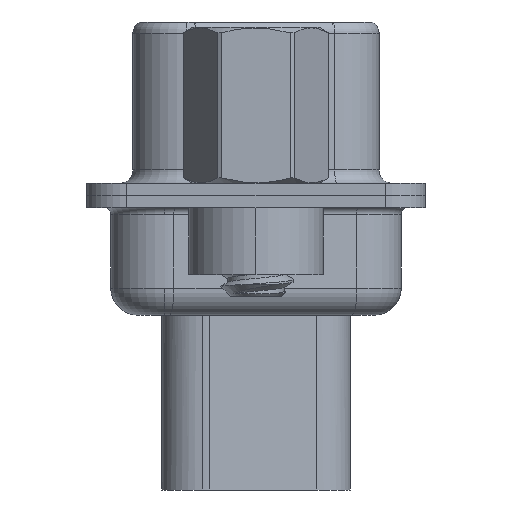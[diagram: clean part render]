
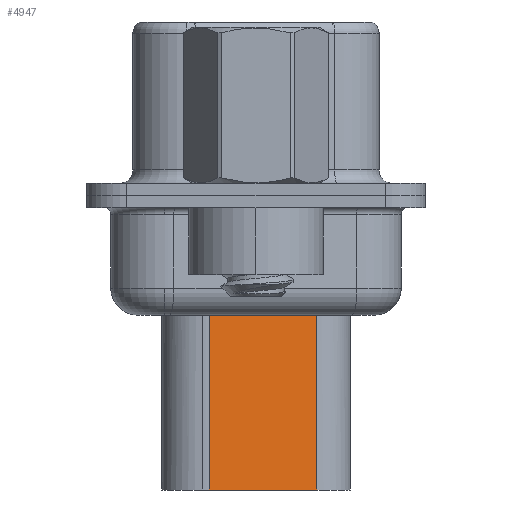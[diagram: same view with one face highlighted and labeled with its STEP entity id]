
A CAD part, left-side view. The second image highlights one B-rep face of the part: STEP entity #4947.
In plain terms, the highlighted planar face has unit normal (-0.985, -0.174, 0).
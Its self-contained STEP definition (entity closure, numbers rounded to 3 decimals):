
#1136 = ORIENTED_EDGE ( 'NONE', *, *, #17670, .F. ) ;
#1139 = LINE ( 'NONE', #17734, #26028 ) ;
#1319 = DIRECTION ( 'NONE',  ( 0.174, -0.985, 0. ) ) ;
#4119 = LINE ( 'NONE', #20710, #21569 ) ;
#4580 = CARTESIAN_POINT ( 'NONE',  ( 5.229, -2.26, -10.95 ) ) ;
#4947 = ADVANCED_FACE ( 'NONE', ( #22006 ), #24309, .T. ) ;
#5405 = EDGE_LOOP ( 'NONE', ( #1136, #11398, #21085, #8418 ) ) ;
#6626 = VECTOR ( 'NONE', #25549, 1000. ) ;
#6658 = CARTESIAN_POINT ( 'NONE',  ( 5.229, -2.26, -3.1 ) ) ;
#7955 = CARTESIAN_POINT ( 'NONE',  ( 4.524, 1.74, -10.95 ) ) ;
#8418 = ORIENTED_EDGE ( 'NONE', *, *, #20001, .F. ) ;
#8926 = AXIS2_PLACEMENT_3D ( 'NONE', #11664, #19960, #1319 ) ;
#9979 = VERTEX_POINT ( 'NONE', #4580 ) ;
#10259 = DIRECTION ( 'NONE',  ( -0.174, 0.985, 0. ) ) ;
#11398 = ORIENTED_EDGE ( 'NONE', *, *, #16700, .T. ) ;
#11664 = CARTESIAN_POINT ( 'NONE',  ( 4.524, 1.74, -3.1 ) ) ;
#13109 = CARTESIAN_POINT ( 'NONE',  ( 5.229, -2.26, -3.975 ) ) ;
#13189 = LINE ( 'NONE', #6658, #6626 ) ;
#13522 = EDGE_CURVE ( 'NONE', #15547, #23128, #1139, .T. ) ;
#15547 = VERTEX_POINT ( 'NONE', #23853 ) ;
#16700 = EDGE_CURVE ( 'NONE', #24675, #15547, #25219, .T. ) ;
#17670 = EDGE_CURVE ( 'NONE', #24675, #9979, #13189, .T. ) ;
#17734 = CARTESIAN_POINT ( 'NONE',  ( 4.524, 1.74, -3.1 ) ) ;
#19233 = DIRECTION ( 'NONE',  ( -0.174, 0.985, 0. ) ) ;
#19960 = DIRECTION ( 'NONE',  ( -0.985, -0.174, 0. ) ) ;
#20001 = EDGE_CURVE ( 'NONE', #9979, #23128, #4119, .T. ) ;
#20710 = CARTESIAN_POINT ( 'NONE',  ( 4.524, 1.74, -10.95 ) ) ;
#21085 = ORIENTED_EDGE ( 'NONE', *, *, #13522, .T. ) ;
#21569 = VECTOR ( 'NONE', #10259, 1000. ) ;
#22006 = FACE_OUTER_BOUND ( 'NONE', #5405, .T. ) ;
#23128 = VERTEX_POINT ( 'NONE', #7955 ) ;
#23853 = CARTESIAN_POINT ( 'NONE',  ( 4.524, 1.74, -3.975 ) ) ;
#24309 = PLANE ( 'NONE',  #8926 ) ;
#24675 = VERTEX_POINT ( 'NONE', #13109 ) ;
#24790 = DIRECTION ( 'NONE',  ( 0., 0., -1. ) ) ;
#25219 = LINE ( 'NONE', #25756, #26641 ) ;
#25549 = DIRECTION ( 'NONE',  ( 0., 0., -1. ) ) ;
#25756 = CARTESIAN_POINT ( 'NONE',  ( 4.353, 2.709, -3.975 ) ) ;
#26028 = VECTOR ( 'NONE', #24790, 1000. ) ;
#26641 = VECTOR ( 'NONE', #19233, 1000. ) ;
